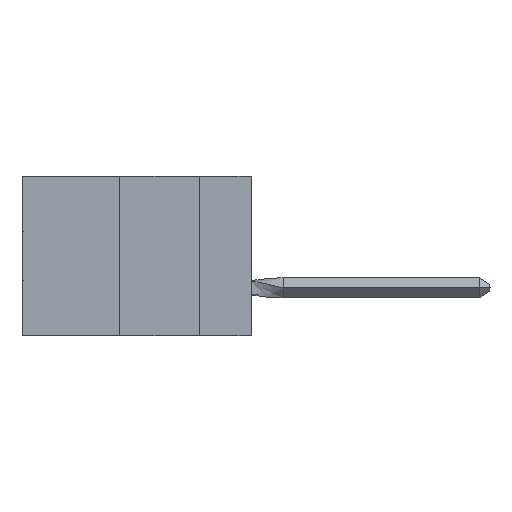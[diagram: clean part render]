
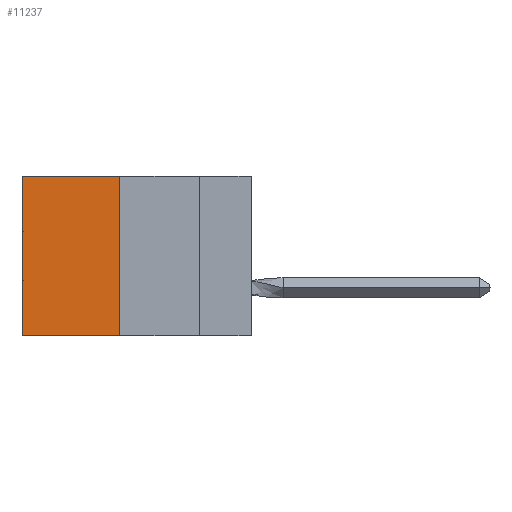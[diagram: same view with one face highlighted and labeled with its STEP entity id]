
A CAD part, left-side view. The second image highlights one B-rep face of the part: STEP entity #11237.
In plain terms, the highlighted planar face has unit normal (-1, 0, 0).
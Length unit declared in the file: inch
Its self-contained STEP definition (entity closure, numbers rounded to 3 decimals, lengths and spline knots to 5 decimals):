
#482 = LINE ( 'NONE', #3137, #16628 ) ;
#2230 = VERTEX_POINT ( 'NONE', #28554 ) ;
#2575 = LINE ( 'NONE', #5736, #26583 ) ;
#3137 = CARTESIAN_POINT ( 'NONE',  ( 0.305, 0.413, -0.5 ) ) ;
#3160 = ORIENTED_EDGE ( 'NONE', *, *, #30522, .T. ) ;
#3365 = LINE ( 'NONE', #9405, #26393 ) ;
#5736 = CARTESIAN_POINT ( 'NONE',  ( 0.305, 0.72, -0.5 ) ) ;
#5884 = AXIS2_PLACEMENT_3D ( 'NONE', #9930, #35223, #13656 ) ;
#6552 = EDGE_CURVE ( 'NONE', #2230, #11093, #482, .T. ) ;
#7578 = DIRECTION ( 'NONE',  ( 0., 1., 0. ) ) ;
#9364 = ORIENTED_EDGE ( 'NONE', *, *, #19464, .T. ) ;
#9405 = CARTESIAN_POINT ( 'NONE',  ( 0.305, 0.413, -0.5 ) ) ;
#9930 = CARTESIAN_POINT ( 'NONE',  ( 0.305, 0.413, -0.5 ) ) ;
#10208 = PLANE ( 'NONE',  #5884 ) ;
#11089 = ORIENTED_EDGE ( 'NONE', *, *, #24841, .F. ) ;
#11093 = VERTEX_POINT ( 'NONE', #37992 ) ;
#11237 = ADVANCED_FACE ( 'NONE', ( #20439 ), #10208, .F. ) ;
#12023 = DIRECTION ( 'NONE',  ( 0., 0., -1. ) ) ;
#12602 = DIRECTION ( 'NONE',  ( 0., 0., -1. ) ) ;
#13245 = ORIENTED_EDGE ( 'NONE', *, *, #6552, .F. ) ;
#13656 = DIRECTION ( 'NONE',  ( 0., 0., -1. ) ) ;
#15010 = CARTESIAN_POINT ( 'NONE',  ( 0.305, 0.72, 0. ) ) ;
#16628 = VECTOR ( 'NONE', #12023, 39.37008 ) ;
#19464 = EDGE_CURVE ( 'NONE', #26360, #29167, #2575, .T. ) ;
#20439 = FACE_OUTER_BOUND ( 'NONE', #38918, .T. ) ;
#23344 = CARTESIAN_POINT ( 'NONE',  ( 0.305, 0.413, 0. ) ) ;
#24841 = EDGE_CURVE ( 'NONE', #11093, #29167, #3365, .T. ) ;
#26360 = VERTEX_POINT ( 'NONE', #15010 ) ;
#26393 = VECTOR ( 'NONE', #28420, 39.37008 ) ;
#26583 = VECTOR ( 'NONE', #12602, 39.37008 ) ;
#28420 = DIRECTION ( 'NONE',  ( 0., 1., 0. ) ) ;
#28554 = CARTESIAN_POINT ( 'NONE',  ( 0.305, 0.413, 0. ) ) ;
#29167 = VERTEX_POINT ( 'NONE', #35367 ) ;
#29823 = LINE ( 'NONE', #23344, #35733 ) ;
#30522 = EDGE_CURVE ( 'NONE', #2230, #26360, #29823, .T. ) ;
#35223 = DIRECTION ( 'NONE',  ( 1., 0., 0. ) ) ;
#35367 = CARTESIAN_POINT ( 'NONE',  ( 0.305, 0.72, -0.5 ) ) ;
#35733 = VECTOR ( 'NONE', #7578, 39.37008 ) ;
#37992 = CARTESIAN_POINT ( 'NONE',  ( 0.305, 0.413, -0.5 ) ) ;
#38918 = EDGE_LOOP ( 'NONE', ( #9364, #11089, #13245, #3160 ) ) ;
